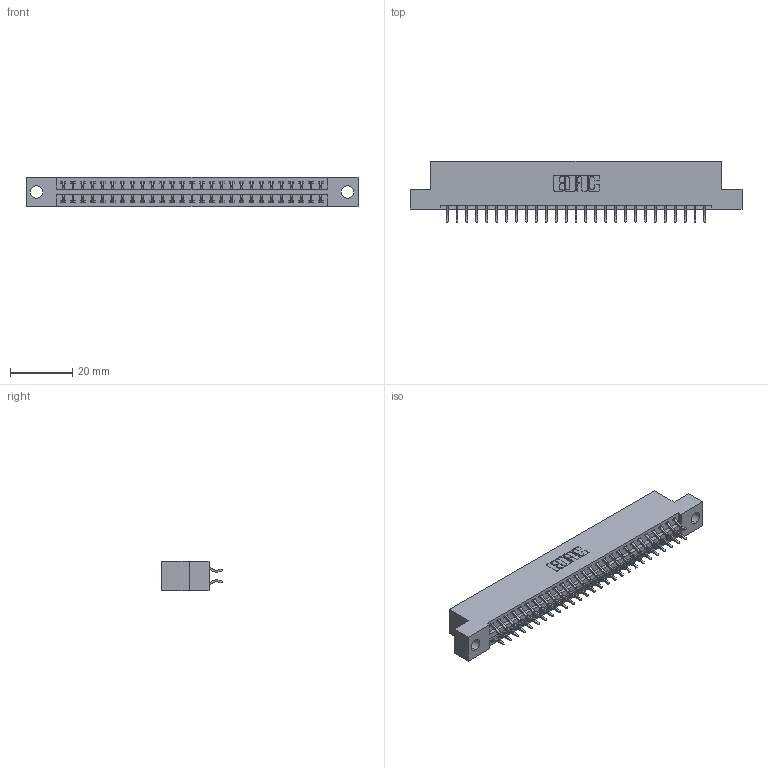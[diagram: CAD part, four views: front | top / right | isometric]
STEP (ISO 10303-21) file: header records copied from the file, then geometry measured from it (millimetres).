
FILE_DESCRIPTION (( 'STEP AP203' ), '1' );
FILE_NAME ('346-054-556-204.STEP', '2022-05-21T04:00:13', ( '' ), ( '' ), 'SwSTEP 2.0', 'SolidWorks 2020', '' );
FILE_SCHEMA (( 'CONFIG_CONTROL_DESIGN' ));
Length unit declared in the file: inch
Products named in the file (3): 346 Part_Flush Mounting Lugs - 0.156 Dia-TH; 346-054-556-204; 345-292-001_556 Tail
Assembly tree (55 placements, depth 2):
  346-054-556-204
    346 Part_Flush Mounting Lugs - 0.156 Dia-TH
    345-292-001_556 Tail  x54
Bounding box: 106.3 x 19.57 x 9.4 mm (x, y, z)
Volume: 10140.9 mm3; surface area: 13501.3 mm2
Topology: 55 solids, 55 shells, 3268 faces, 9707 edges, 6398 vertices
Faces by surface type: plane 2196, cylinder 1072
Entity records: 20279 total; most frequent: CARTESIAN_POINT 3382, ORIENTED_EDGE 3302, DIRECTION 3019, EDGE_CURVE 1651, VECTOR 1403, LINE 1403, VERTEX_POINT 1098, AXIS2_PLACEMENT_3D 808
